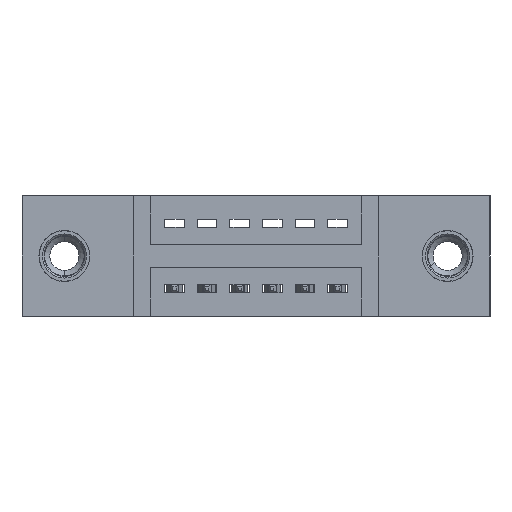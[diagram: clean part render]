
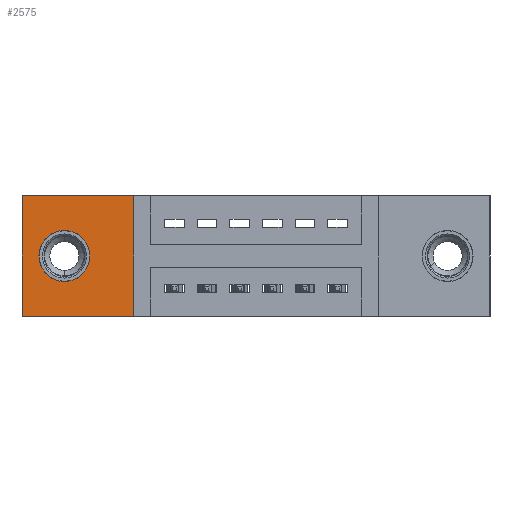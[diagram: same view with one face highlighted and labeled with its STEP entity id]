
A CAD part, front view. The second image highlights one B-rep face of the part: STEP entity #2575.
In plain terms, the highlighted planar face has unit normal (0, -1, 0).
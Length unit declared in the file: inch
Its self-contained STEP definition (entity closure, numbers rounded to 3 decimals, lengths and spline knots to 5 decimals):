
#97 = CARTESIAN_POINT ( 'NONE',  ( 0.13, 0.17, -0.263 ) ) ;
#130 = EDGE_LOOP ( 'NONE', ( #3433, #3270, #1501, #4769 ) ) ;
#501 = EDGE_LOOP ( 'NONE', ( #4923, #1472 ) ) ;
#708 = AXIS2_PLACEMENT_3D ( 'NONE', #2621, #1012, #4324 ) ;
#753 = DIRECTION ( 'NONE',  ( 1., 0., 0. ) ) ;
#1012 = DIRECTION ( 'NONE',  ( 0., -1., 0. ) ) ;
#1030 = DIRECTION ( 'NONE',  ( 0., -1., 0. ) ) ;
#1202 = CARTESIAN_POINT ( 'NONE',  ( 0.3425, 0.17, -0.37 ) ) ;
#1211 = VECTOR ( 'NONE', #10122, 39.37008 ) ;
#1472 = ORIENTED_EDGE ( 'NONE', *, *, #9365, .F. ) ;
#1501 = ORIENTED_EDGE ( 'NONE', *, *, #4659, .T. ) ;
#1898 = CARTESIAN_POINT ( 'NONE',  ( 0., 0.17, -0.37 ) ) ;
#2028 = AXIS2_PLACEMENT_3D ( 'NONE', #10240, #1030, #6135 ) ;
#2116 = CARTESIAN_POINT ( 'NONE',  ( 0., 0.17, 0. ) ) ;
#2159 = CARTESIAN_POINT ( 'NONE',  ( 0.13, 0.17, -0.107 ) ) ;
#2575 = ADVANCED_FACE ( 'NONE', ( #9835, #8661 ), #5602, .T. ) ;
#2621 = CARTESIAN_POINT ( 'NONE',  ( 0.13, 0.17, -0.185 ) ) ;
#3057 = DIRECTION ( 'NONE',  ( 0., -1., 0. ) ) ;
#3270 = ORIENTED_EDGE ( 'NONE', *, *, #8411, .T. ) ;
#3433 = ORIENTED_EDGE ( 'NONE', *, *, #9806, .T. ) ;
#3593 = LINE ( 'NONE', #4883, #7036 ) ;
#3721 = CARTESIAN_POINT ( 'NONE',  ( 0.3425, 0.17, 0. ) ) ;
#3876 = EDGE_CURVE ( 'NONE', #10341, #10400, #5606, .T. ) ;
#4324 = DIRECTION ( 'NONE',  ( 0., 0., -1. ) ) ;
#4659 = EDGE_CURVE ( 'NONE', #10273, #10341, #7513, .T. ) ;
#4729 = VECTOR ( 'NONE', #10416, 39.37008 ) ;
#4769 = ORIENTED_EDGE ( 'NONE', *, *, #3876, .T. ) ;
#4883 = CARTESIAN_POINT ( 'NONE',  ( 0., 0.17, -0.37 ) ) ;
#4923 = ORIENTED_EDGE ( 'NONE', *, *, #7378, .F. ) ;
#5393 = CIRCLE ( 'NONE', #708, 0.078 ) ;
#5532 = CARTESIAN_POINT ( 'NONE',  ( 0., 0.17, 0. ) ) ;
#5602 = PLANE ( 'NONE',  #7837 ) ;
#5606 = LINE ( 'NONE', #5633, #8157 ) ;
#5631 = LINE ( 'NONE', #2116, #4729 ) ;
#5633 = CARTESIAN_POINT ( 'NONE',  ( 0., 0.17, 0. ) ) ;
#6135 = DIRECTION ( 'NONE',  ( 0., 0., -1. ) ) ;
#6318 = VERTEX_POINT ( 'NONE', #1898 ) ;
#6354 = DIRECTION ( 'NONE',  ( 0., 0., -1. ) ) ;
#6422 = CARTESIAN_POINT ( 'NONE',  ( 0., 0.17, -0.37 ) ) ;
#7036 = VECTOR ( 'NONE', #753, 39.37008 ) ;
#7378 = EDGE_CURVE ( 'NONE', #9094, #8757, #10044, .T. ) ;
#7509 = CARTESIAN_POINT ( 'NONE',  ( 0.3425, 0.17, 0. ) ) ;
#7513 = LINE ( 'NONE', #7509, #1211 ) ;
#7837 = AXIS2_PLACEMENT_3D ( 'NONE', #6422, #3057, #6354 ) ;
#8157 = VECTOR ( 'NONE', #9034, 39.37008 ) ;
#8411 = EDGE_CURVE ( 'NONE', #6318, #10273, #3593, .T. ) ;
#8661 = FACE_OUTER_BOUND ( 'NONE', #130, .T. ) ;
#8757 = VERTEX_POINT ( 'NONE', #97 ) ;
#9034 = DIRECTION ( 'NONE',  ( -1., 0., 0. ) ) ;
#9094 = VERTEX_POINT ( 'NONE', #2159 ) ;
#9365 = EDGE_CURVE ( 'NONE', #8757, #9094, #5393, .T. ) ;
#9806 = EDGE_CURVE ( 'NONE', #10400, #6318, #5631, .T. ) ;
#9835 = FACE_BOUND ( 'NONE', #501, .T. ) ;
#10044 = CIRCLE ( 'NONE', #2028, 0.078 ) ;
#10122 = DIRECTION ( 'NONE',  ( 0., 0., 1. ) ) ;
#10240 = CARTESIAN_POINT ( 'NONE',  ( 0.13, 0.17, -0.185 ) ) ;
#10273 = VERTEX_POINT ( 'NONE', #1202 ) ;
#10341 = VERTEX_POINT ( 'NONE', #3721 ) ;
#10400 = VERTEX_POINT ( 'NONE', #5532 ) ;
#10416 = DIRECTION ( 'NONE',  ( 0., 0., -1. ) ) ;
